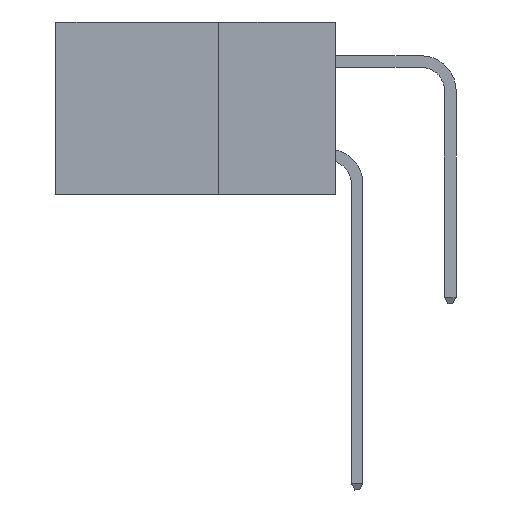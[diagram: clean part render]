
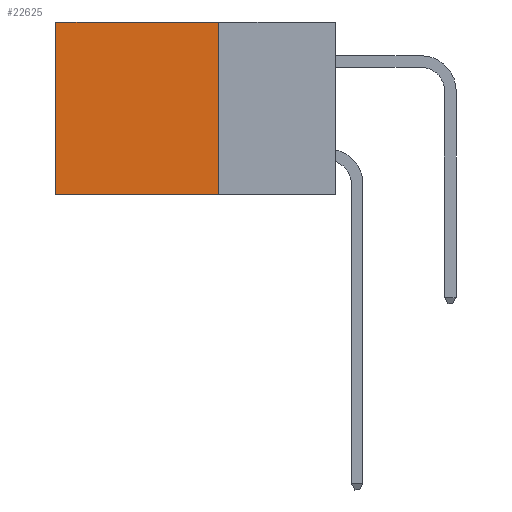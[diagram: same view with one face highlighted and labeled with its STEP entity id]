
A CAD part, left-side view. The second image highlights one B-rep face of the part: STEP entity #22625.
In plain terms, the highlighted planar face has unit normal (-1, 0, 0).
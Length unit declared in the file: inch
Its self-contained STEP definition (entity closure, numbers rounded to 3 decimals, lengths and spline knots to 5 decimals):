
#1835 = PLANE ( 'NONE',  #3308 ) ;
#3308 = AXIS2_PLACEMENT_3D ( 'NONE', #20418, #27440, #13490 ) ;
#3333 = CARTESIAN_POINT ( 'NONE',  ( 0.2875, 0.25, -0.37 ) ) ;
#3921 = VECTOR ( 'NONE', #19611, 39.37008 ) ;
#6092 = ORIENTED_EDGE ( 'NONE', *, *, #16552, .F. ) ;
#7431 = EDGE_LOOP ( 'NONE', ( #9819, #16448, #6092, #14906 ) ) ;
#8813 = DIRECTION ( 'NONE',  ( 0., 1., 0. ) ) ;
#9241 = VECTOR ( 'NONE', #8813, 39.37008 ) ;
#9774 = DIRECTION ( 'NONE',  ( 0., 0., -1. ) ) ;
#9819 = ORIENTED_EDGE ( 'NONE', *, *, #26850, .T. ) ;
#10493 = LINE ( 'NONE', #15617, #22869 ) ;
#10760 = VECTOR ( 'NONE', #9774, 39.37008 ) ;
#11382 = VERTEX_POINT ( 'NONE', #13978 ) ;
#12101 = CARTESIAN_POINT ( 'NONE',  ( 0.2875, 0.25, 0. ) ) ;
#12749 = VERTEX_POINT ( 'NONE', #27049 ) ;
#13371 = CARTESIAN_POINT ( 'NONE',  ( 0.2875, 0.25, 0. ) ) ;
#13490 = DIRECTION ( 'NONE',  ( 0., 0., -1. ) ) ;
#13549 = VERTEX_POINT ( 'NONE', #27532 ) ;
#13978 = CARTESIAN_POINT ( 'NONE',  ( 0.2875, 0.25, 0. ) ) ;
#14906 = ORIENTED_EDGE ( 'NONE', *, *, #17484, .T. ) ;
#15245 = EDGE_CURVE ( 'NONE', #16666, #12749, #16314, .T. ) ;
#15617 = CARTESIAN_POINT ( 'NONE',  ( 0.2875, 0.6, 0. ) ) ;
#16314 = LINE ( 'NONE', #3333, #3921 ) ;
#16448 = ORIENTED_EDGE ( 'NONE', *, *, #15245, .F. ) ;
#16552 = EDGE_CURVE ( 'NONE', #11382, #16666, #29311, .T. ) ;
#16666 = VERTEX_POINT ( 'NONE', #17605 ) ;
#16897 = FACE_OUTER_BOUND ( 'NONE', #7431, .T. ) ;
#17484 = EDGE_CURVE ( 'NONE', #11382, #13549, #21615, .T. ) ;
#17605 = CARTESIAN_POINT ( 'NONE',  ( 0.2875, 0.25, -0.37 ) ) ;
#19611 = DIRECTION ( 'NONE',  ( 0., 1., 0. ) ) ;
#20418 = CARTESIAN_POINT ( 'NONE',  ( 0.2875, 0.25, 0. ) ) ;
#21615 = LINE ( 'NONE', #13371, #9241 ) ;
#22625 = ADVANCED_FACE ( 'NONE', ( #16897 ), #1835, .F. ) ;
#22869 = VECTOR ( 'NONE', #27194, 39.37008 ) ;
#26850 = EDGE_CURVE ( 'NONE', #13549, #12749, #10493, .T. ) ;
#27049 = CARTESIAN_POINT ( 'NONE',  ( 0.2875, 0.6, -0.37 ) ) ;
#27194 = DIRECTION ( 'NONE',  ( 0., 0., -1. ) ) ;
#27440 = DIRECTION ( 'NONE',  ( 1., 0., 0. ) ) ;
#27532 = CARTESIAN_POINT ( 'NONE',  ( 0.2875, 0.6, 0. ) ) ;
#29311 = LINE ( 'NONE', #12101, #10760 ) ;
